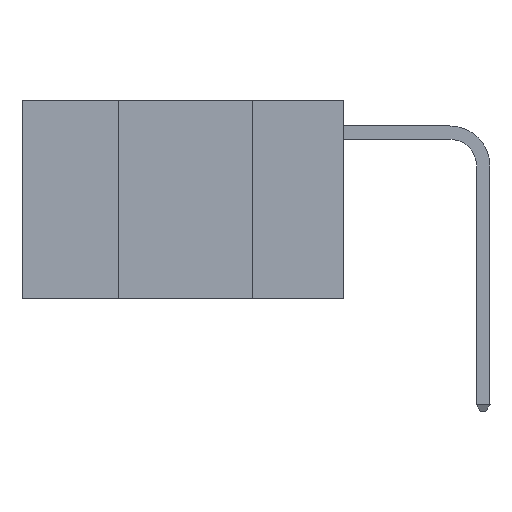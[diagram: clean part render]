
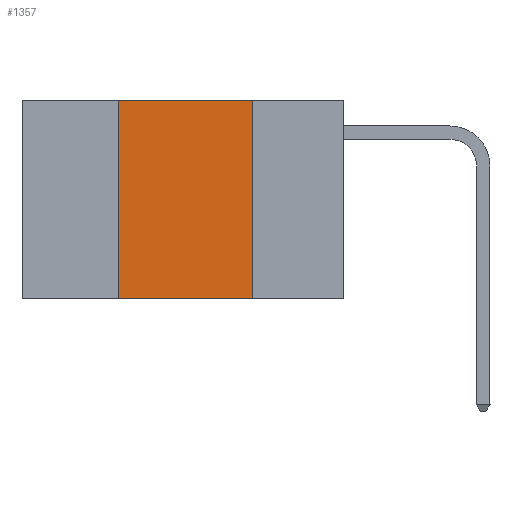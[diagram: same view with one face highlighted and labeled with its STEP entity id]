
A CAD part, left-side view. The second image highlights one B-rep face of the part: STEP entity #1357.
In plain terms, the highlighted planar face has unit normal (-1, 0, 0).
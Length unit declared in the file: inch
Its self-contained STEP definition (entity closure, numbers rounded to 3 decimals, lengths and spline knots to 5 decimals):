
#444 = VECTOR ( 'NONE', #6004, 39.37008 ) ;
#687 = VERTEX_POINT ( 'NONE', #2884 ) ;
#1053 = PLANE ( 'NONE',  #5273 ) ;
#1125 = EDGE_CURVE ( 'NONE', #4529, #4971, #1554, .T. ) ;
#1357 = ADVANCED_FACE ( 'NONE', ( #8566 ), #1053, .F. ) ;
#1400 = EDGE_CURVE ( 'NONE', #3595, #687, #5600, .T. ) ;
#1554 = LINE ( 'NONE', #7836, #444 ) ;
#1571 = DIRECTION ( 'NONE',  ( 0., -1., 0. ) ) ;
#1811 = CARTESIAN_POINT ( 'NONE',  ( 0., 0.6, 0. ) ) ;
#1873 = EDGE_LOOP ( 'NONE', ( #8549, #5411, #5406, #9116 ) ) ;
#2278 = DIRECTION ( 'NONE',  ( 0., 0., -1. ) ) ;
#2488 = EDGE_CURVE ( 'NONE', #4529, #687, #7019, .T. ) ;
#2884 = CARTESIAN_POINT ( 'NONE',  ( 0., 0.17, -0.37 ) ) ;
#3315 = CARTESIAN_POINT ( 'NONE',  ( 0., 0.6, 0. ) ) ;
#3595 = VERTEX_POINT ( 'NONE', #6330 ) ;
#3725 = DIRECTION ( 'NONE',  ( 1., 0., 0. ) ) ;
#3750 = DIRECTION ( 'NONE',  ( 0., 0., -1. ) ) ;
#4529 = VERTEX_POINT ( 'NONE', #9144 ) ;
#4971 = VERTEX_POINT ( 'NONE', #9049 ) ;
#5273 = AXIS2_PLACEMENT_3D ( 'NONE', #3315, #3725, #3750 ) ;
#5406 = ORIENTED_EDGE ( 'NONE', *, *, #1125, .F. ) ;
#5411 = ORIENTED_EDGE ( 'NONE', *, *, #7531, .F. ) ;
#5434 = DIRECTION ( 'NONE',  ( 0., -1., 0. ) ) ;
#5516 = VECTOR ( 'NONE', #1571, 39.37008 ) ;
#5592 = VECTOR ( 'NONE', #2278, 39.37008 ) ;
#5600 = LINE ( 'NONE', #9056, #5592 ) ;
#5787 = LINE ( 'NONE', #1811, #5516 ) ;
#6004 = DIRECTION ( 'NONE',  ( 0., 0., 1. ) ) ;
#6330 = CARTESIAN_POINT ( 'NONE',  ( 0., 0.17, 0. ) ) ;
#6540 = VECTOR ( 'NONE', #5434, 39.37008 ) ;
#7019 = LINE ( 'NONE', #8277, #6540 ) ;
#7531 = EDGE_CURVE ( 'NONE', #4971, #3595, #5787, .T. ) ;
#7836 = CARTESIAN_POINT ( 'NONE',  ( 0., 0.42, 0. ) ) ;
#8277 = CARTESIAN_POINT ( 'NONE',  ( 0., 0.6, -0.37 ) ) ;
#8549 = ORIENTED_EDGE ( 'NONE', *, *, #1400, .F. ) ;
#8566 = FACE_OUTER_BOUND ( 'NONE', #1873, .T. ) ;
#9049 = CARTESIAN_POINT ( 'NONE',  ( 0., 0.42, 0. ) ) ;
#9056 = CARTESIAN_POINT ( 'NONE',  ( 0., 0.17, 0. ) ) ;
#9116 = ORIENTED_EDGE ( 'NONE', *, *, #2488, .T. ) ;
#9144 = CARTESIAN_POINT ( 'NONE',  ( 0., 0.42, -0.37 ) ) ;
